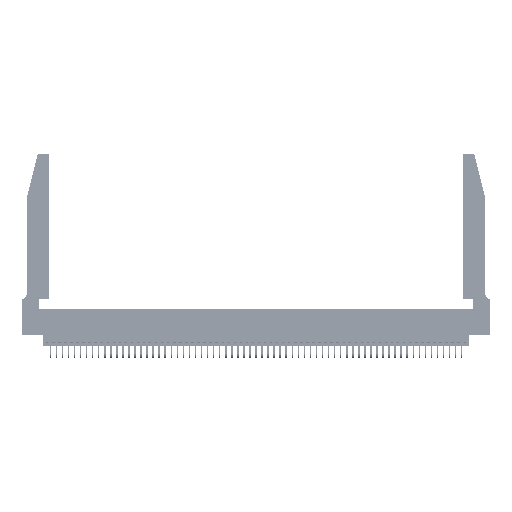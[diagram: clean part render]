
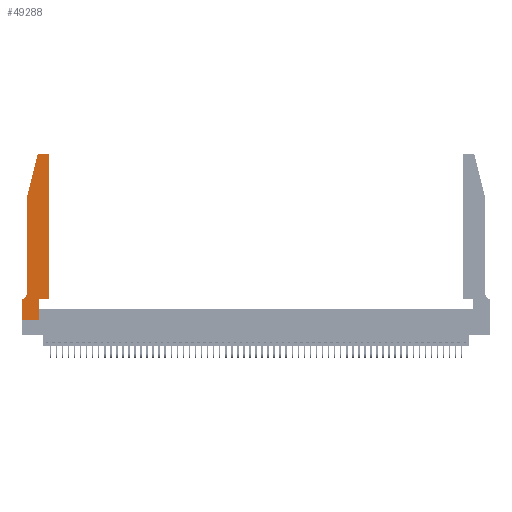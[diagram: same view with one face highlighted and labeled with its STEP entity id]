
A CAD part, top view. The second image highlights one B-rep face of the part: STEP entity #49288.
In plain terms, the highlighted planar face has unit normal (0, 0, 1).
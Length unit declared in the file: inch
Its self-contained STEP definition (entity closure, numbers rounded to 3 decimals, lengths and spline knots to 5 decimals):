
#333 = EDGE_CURVE ( 'NONE', #32498, #1722, #47329, .T. ) ;
#1566 = EDGE_CURVE ( 'NONE', #25542, #28124, #14306, .T. ) ;
#1697 = CARTESIAN_POINT ( 'NONE',  ( 0.2865, 0.35, 0.37 ) ) ;
#1722 = VERTEX_POINT ( 'NONE', #33326 ) ;
#2557 = CARTESIAN_POINT ( 'NONE',  ( 0., 0., 0.37 ) ) ;
#3737 = VERTEX_POINT ( 'NONE', #7568 ) ;
#5359 = DIRECTION ( 'NONE',  ( 1., 0., 0. ) ) ;
#5698 = ORIENTED_EDGE ( 'NONE', *, *, #12879, .T. ) ;
#6538 = CARTESIAN_POINT ( 'NONE',  ( 0., 0., 0.37 ) ) ;
#7306 = VECTOR ( 'NONE', #19072, 39.37008 ) ;
#7568 = CARTESIAN_POINT ( 'NONE',  ( 0.2865, 0., 0.37 ) ) ;
#8086 = VERTEX_POINT ( 'NONE', #52483 ) ;
#8253 = FACE_OUTER_BOUND ( 'NONE', #10758, .T. ) ;
#8812 = EDGE_CURVE ( 'NONE', #28124, #22973, #29925, .T. ) ;
#9440 = DIRECTION ( 'NONE',  ( 0., 0., -1. ) ) ;
#9597 = VERTEX_POINT ( 'NONE', #48492 ) ;
#10239 = DIRECTION ( 'NONE',  ( 0., 1., 0. ) ) ;
#10327 = CARTESIAN_POINT ( 'NONE',  ( 0.4505, 0.35, 0.37 ) ) ;
#10758 = EDGE_LOOP ( 'NONE', ( #47220, #19025, #11964, #16026, #47448, #22603, #19677, #43400, #5698, #22721, #49201, #13324 ) ) ;
#11568 = CARTESIAN_POINT ( 'NONE',  ( 0.284, 2.75, 0.37 ) ) ;
#11964 = ORIENTED_EDGE ( 'NONE', *, *, #12576, .T. ) ;
#12576 = EDGE_CURVE ( 'NONE', #9597, #8086, #46040, .T. ) ;
#12879 = EDGE_CURVE ( 'NONE', #3737, #25595, #32259, .T. ) ;
#13324 = ORIENTED_EDGE ( 'NONE', *, *, #1566, .T. ) ;
#14306 = CIRCLE ( 'NONE', #16791, 0.03 ) ;
#14513 = CARTESIAN_POINT ( 'NONE',  ( 0.4205, 2.72, 0.37 ) ) ;
#14592 = CARTESIAN_POINT ( 'NONE',  ( 0.0755, 0.35, 0.37 ) ) ;
#15281 = DIRECTION ( 'NONE',  ( 1., 0., 0. ) ) ;
#16026 = ORIENTED_EDGE ( 'NONE', *, *, #54815, .T. ) ;
#16524 = EDGE_CURVE ( 'NONE', #39970, #3737, #25577, .T. ) ;
#16594 = DIRECTION ( 'NONE',  ( 0., -1., 0. ) ) ;
#16791 = AXIS2_PLACEMENT_3D ( 'NONE', #14513, #40997, #50278 ) ;
#16883 = CARTESIAN_POINT ( 'NONE',  ( 0., 0.35, 0.37 ) ) ;
#19025 = ORIENTED_EDGE ( 'NONE', *, *, #43323, .T. ) ;
#19072 = DIRECTION ( 'NONE',  ( 0., -1., 0. ) ) ;
#19677 = ORIENTED_EDGE ( 'NONE', *, *, #53987, .T. ) ;
#20076 = AXIS2_PLACEMENT_3D ( 'NONE', #26716, #31519, #5359 ) ;
#20733 = CARTESIAN_POINT ( 'NONE',  ( 0.4505, 0.35, 0.37 ) ) ;
#20804 = VECTOR ( 'NONE', #31023, 39.37008 ) ;
#21590 = EDGE_CURVE ( 'NONE', #1722, #27615, #28330, .T. ) ;
#21740 = CARTESIAN_POINT ( 'NONE',  ( 0.0755, 0.42, 0.37 ) ) ;
#21776 = LINE ( 'NONE', #6538, #7306 ) ;
#22603 = ORIENTED_EDGE ( 'NONE', *, *, #21590, .T. ) ;
#22721 = ORIENTED_EDGE ( 'NONE', *, *, #28131, .T. ) ;
#22973 = VERTEX_POINT ( 'NONE', #11568 ) ;
#25542 = VERTEX_POINT ( 'NONE', #50563 ) ;
#25577 = LINE ( 'NONE', #53570, #20804 ) ;
#25595 = VERTEX_POINT ( 'NONE', #45733 ) ;
#26716 = CARTESIAN_POINT ( 'NONE',  ( 0., 0.35, 0.37 ) ) ;
#27595 = VERTEX_POINT ( 'NONE', #20733 ) ;
#27615 = VERTEX_POINT ( 'NONE', #16883 ) ;
#27882 = VECTOR ( 'NONE', #39304, 39.37008 ) ;
#28124 = VERTEX_POINT ( 'NONE', #32781 ) ;
#28131 = EDGE_CURVE ( 'NONE', #25595, #27595, #29400, .T. ) ;
#28330 = LINE ( 'NONE', #14592, #53141 ) ;
#29149 = DIRECTION ( 'NONE',  ( 1., 0., 0. ) ) ;
#29400 = LINE ( 'NONE', #10327, #48019 ) ;
#29848 = DIRECTION ( 'NONE',  ( -0.239, -0.971, 0. ) ) ;
#29925 = LINE ( 'NONE', #56875, #27882 ) ;
#30792 = VECTOR ( 'NONE', #56836, 39.37008 ) ;
#31023 = DIRECTION ( 'NONE',  ( 1., 0., 0. ) ) ;
#31519 = DIRECTION ( 'NONE',  ( 0., 0., 1. ) ) ;
#31882 = EDGE_CURVE ( 'NONE', #27595, #25542, #42485, .T. ) ;
#32259 = LINE ( 'NONE', #1697, #35680 ) ;
#32498 = VERTEX_POINT ( 'NONE', #21740 ) ;
#32781 = CARTESIAN_POINT ( 'NONE',  ( 0.4205, 2.75, 0.37 ) ) ;
#33326 = CARTESIAN_POINT ( 'NONE',  ( 0.0055, 0.35, 0.37 ) ) ;
#34162 = DIRECTION ( 'NONE',  ( 0., 0., 1. ) ) ;
#35680 = VECTOR ( 'NONE', #10239, 39.37008 ) ;
#35768 = PLANE ( 'NONE',  #20076 ) ;
#37469 = LINE ( 'NONE', #56606, #43708 ) ;
#39304 = DIRECTION ( 'NONE',  ( -1., 0., 0. ) ) ;
#39613 = CARTESIAN_POINT ( 'NONE',  ( 0.0055, 0.42, 0.37 ) ) ;
#39970 = VERTEX_POINT ( 'NONE', #2557 ) ;
#40158 = DIRECTION ( 'NONE',  ( -1., 0., 0. ) ) ;
#40997 = DIRECTION ( 'NONE',  ( 0., 0., 1. ) ) ;
#41734 = AXIS2_PLACEMENT_3D ( 'NONE', #39613, #9440, #40158 ) ;
#42485 = LINE ( 'NONE', #52758, #30792 ) ;
#43323 = EDGE_CURVE ( 'NONE', #22973, #9597, #54668, .T. ) ;
#43400 = ORIENTED_EDGE ( 'NONE', *, *, #16524, .T. ) ;
#43708 = VECTOR ( 'NONE', #16594, 39.37008 ) ;
#45134 = DIRECTION ( 'NONE',  ( -1., 0., 0. ) ) ;
#45733 = CARTESIAN_POINT ( 'NONE',  ( 0.2865, 0.35, 0.37 ) ) ;
#46040 = LINE ( 'NONE', #52168, #47430 ) ;
#47220 = ORIENTED_EDGE ( 'NONE', *, *, #8812, .T. ) ;
#47329 = CIRCLE ( 'NONE', #41734, 0.07 ) ;
#47430 = VECTOR ( 'NONE', #29848, 39.37008 ) ;
#47448 = ORIENTED_EDGE ( 'NONE', *, *, #333, .T. ) ;
#48019 = VECTOR ( 'NONE', #15281, 39.37008 ) ;
#48492 = CARTESIAN_POINT ( 'NONE',  ( 0.25487, 2.72718, 0.37 ) ) ;
#48647 = AXIS2_PLACEMENT_3D ( 'NONE', #51291, #34162, #29149 ) ;
#49201 = ORIENTED_EDGE ( 'NONE', *, *, #31882, .T. ) ;
#49288 = ADVANCED_FACE ( 'NONE', ( #8253 ), #35768, .T. ) ;
#50278 = DIRECTION ( 'NONE',  ( 1., 0., 0. ) ) ;
#50563 = CARTESIAN_POINT ( 'NONE',  ( 0.4505, 2.72, 0.37 ) ) ;
#51291 = CARTESIAN_POINT ( 'NONE',  ( 0.284, 2.72, 0.37 ) ) ;
#52168 = CARTESIAN_POINT ( 'NONE',  ( 0.0755, 2., 0.37 ) ) ;
#52483 = CARTESIAN_POINT ( 'NONE',  ( 0.0755, 2., 0.37 ) ) ;
#52758 = CARTESIAN_POINT ( 'NONE',  ( 0.4505, 0.35, 0.37 ) ) ;
#53141 = VECTOR ( 'NONE', #45134, 39.37008 ) ;
#53570 = CARTESIAN_POINT ( 'NONE',  ( 0., 0., 0.37 ) ) ;
#53987 = EDGE_CURVE ( 'NONE', #27615, #39970, #21776, .T. ) ;
#54668 = CIRCLE ( 'NONE', #48647, 0.03 ) ;
#54815 = EDGE_CURVE ( 'NONE', #8086, #32498, #37469, .T. ) ;
#56606 = CARTESIAN_POINT ( 'NONE',  ( 0.0755, 2., 0.37 ) ) ;
#56836 = DIRECTION ( 'NONE',  ( 0., 1., 0. ) ) ;
#56875 = CARTESIAN_POINT ( 'NONE',  ( 0.2605, 2.75, 0.37 ) ) ;
